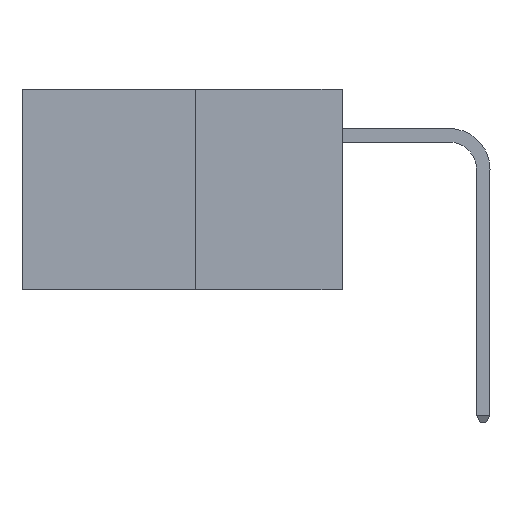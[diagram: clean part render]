
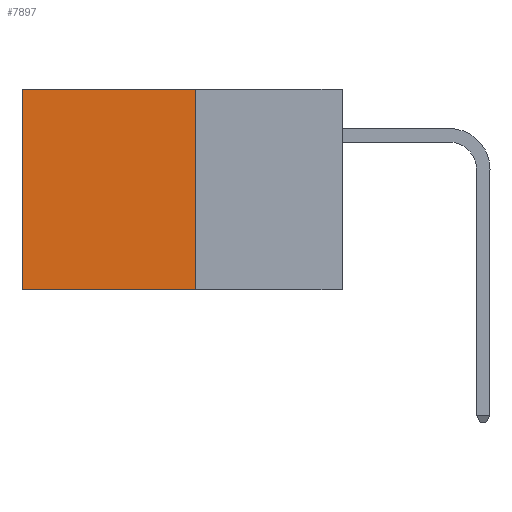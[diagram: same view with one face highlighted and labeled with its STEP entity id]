
A CAD part, left-side view. The second image highlights one B-rep face of the part: STEP entity #7897.
In plain terms, the highlighted planar face has unit normal (-1, 0, 0).
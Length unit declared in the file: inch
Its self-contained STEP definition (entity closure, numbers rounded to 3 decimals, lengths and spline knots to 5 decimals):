
#37 = CARTESIAN_POINT ( 'NONE',  ( 0.277, 0.27, 0. ) ) ;
#382 = FACE_OUTER_BOUND ( 'NONE', #7261, .T. ) ;
#566 = CARTESIAN_POINT ( 'NONE',  ( 0.277, 0.27, -0.37 ) ) ;
#1604 = CARTESIAN_POINT ( 'NONE',  ( 0.277, 0.59, 0. ) ) ;
#1617 = ORIENTED_EDGE ( 'NONE', *, *, #12190, .F. ) ;
#2531 = VECTOR ( 'NONE', #15168, 39.37008 ) ;
#2862 = LINE ( 'NONE', #7197, #3271 ) ;
#3271 = VECTOR ( 'NONE', #7107, 39.37008 ) ;
#3276 = DIRECTION ( 'NONE',  ( 0., 0., -1. ) ) ;
#3613 = EDGE_CURVE ( 'NONE', #11918, #7604, #2862, .T. ) ;
#5315 = EDGE_CURVE ( 'NONE', #14119, #7604, #13955, .T. ) ;
#5334 = CARTESIAN_POINT ( 'NONE',  ( 0.277, 0.59, -0.37 ) ) ;
#5393 = AXIS2_PLACEMENT_3D ( 'NONE', #566, #11206, #3276 ) ;
#6930 = VECTOR ( 'NONE', #14734, 39.37008 ) ;
#7107 = DIRECTION ( 'NONE',  ( 0., 1., 0. ) ) ;
#7197 = CARTESIAN_POINT ( 'NONE',  ( 0.277, 0.27, -0.37 ) ) ;
#7261 = EDGE_LOOP ( 'NONE', ( #8939, #10421, #1617, #16182 ) ) ;
#7604 = VERTEX_POINT ( 'NONE', #5334 ) ;
#7638 = VERTEX_POINT ( 'NONE', #37 ) ;
#7897 = ADVANCED_FACE ( 'NONE', ( #382 ), #8567, .F. ) ;
#8180 = CARTESIAN_POINT ( 'NONE',  ( 0.277, 0.59, -0.37 ) ) ;
#8567 = PLANE ( 'NONE',  #5393 ) ;
#8812 = LINE ( 'NONE', #10611, #12288 ) ;
#8939 = ORIENTED_EDGE ( 'NONE', *, *, #5315, .T. ) ;
#10421 = ORIENTED_EDGE ( 'NONE', *, *, #3613, .F. ) ;
#10611 = CARTESIAN_POINT ( 'NONE',  ( 0.277, 0.27, -0.37 ) ) ;
#11206 = DIRECTION ( 'NONE',  ( 1., 0., 0. ) ) ;
#11918 = VERTEX_POINT ( 'NONE', #14012 ) ;
#12190 = EDGE_CURVE ( 'NONE', #7638, #11918, #8812, .T. ) ;
#12288 = VECTOR ( 'NONE', #17179, 39.37008 ) ;
#13058 = LINE ( 'NONE', #16438, #2531 ) ;
#13955 = LINE ( 'NONE', #8180, #6930 ) ;
#14012 = CARTESIAN_POINT ( 'NONE',  ( 0.277, 0.27, -0.37 ) ) ;
#14119 = VERTEX_POINT ( 'NONE', #1604 ) ;
#14294 = EDGE_CURVE ( 'NONE', #7638, #14119, #13058, .T. ) ;
#14734 = DIRECTION ( 'NONE',  ( 0., 0., -1. ) ) ;
#15168 = DIRECTION ( 'NONE',  ( 0., 1., 0. ) ) ;
#16182 = ORIENTED_EDGE ( 'NONE', *, *, #14294, .T. ) ;
#16438 = CARTESIAN_POINT ( 'NONE',  ( 0.277, 0.27, 0. ) ) ;
#17179 = DIRECTION ( 'NONE',  ( 0., 0., -1. ) ) ;
